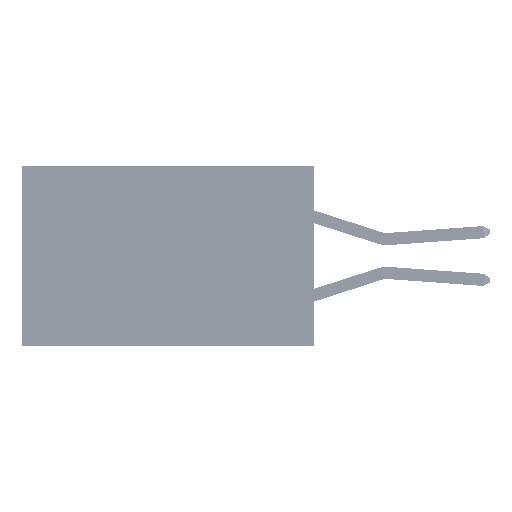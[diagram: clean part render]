
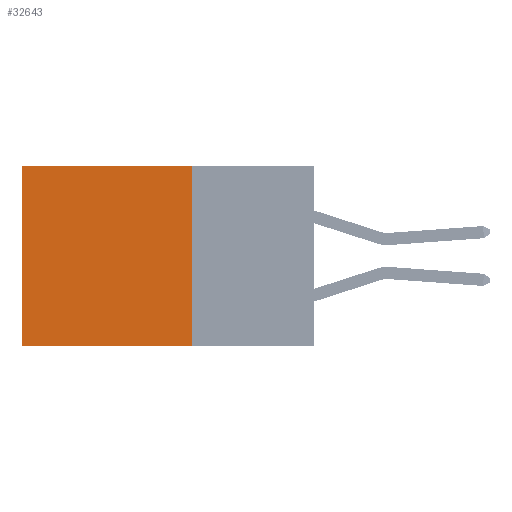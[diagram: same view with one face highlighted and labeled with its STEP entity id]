
A CAD part, left-side view. The second image highlights one B-rep face of the part: STEP entity #32643.
In plain terms, the highlighted planar face has unit normal (-1, 0, 0).
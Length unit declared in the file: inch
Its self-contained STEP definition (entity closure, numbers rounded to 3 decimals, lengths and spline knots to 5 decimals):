
#1590 = EDGE_CURVE ( 'NONE', #46278, #43713, #3092, .T. ) ;
#3092 = LINE ( 'NONE', #15803, #29588 ) ;
#3892 = FACE_OUTER_BOUND ( 'NONE', #48958, .T. ) ;
#6609 = DIRECTION ( 'NONE',  ( 0., 0., -1. ) ) ;
#9017 = VECTOR ( 'NONE', #17560, 39.37008 ) ;
#15061 = LINE ( 'NONE', #21394, #9017 ) ;
#15562 = DIRECTION ( 'NONE',  ( 0., 1., 0. ) ) ;
#15803 = CARTESIAN_POINT ( 'NONE',  ( 0.2875, 0.25, 0. ) ) ;
#15960 = CARTESIAN_POINT ( 'NONE',  ( 0.2875, 0.25, -0.37 ) ) ;
#17560 = DIRECTION ( 'NONE',  ( 0., 1., 0. ) ) ;
#19490 = DIRECTION ( 'NONE',  ( 0., 0., -1. ) ) ;
#20014 = ORIENTED_EDGE ( 'NONE', *, *, #42223, .T. ) ;
#20800 = VECTOR ( 'NONE', #15562, 39.37008 ) ;
#21354 = LINE ( 'NONE', #31228, #37404 ) ;
#21394 = CARTESIAN_POINT ( 'NONE',  ( 0.2875, 0.25, -0.37 ) ) ;
#27652 = CARTESIAN_POINT ( 'NONE',  ( 0.2875, 0.25, 0. ) ) ;
#29588 = VECTOR ( 'NONE', #38997, 39.37008 ) ;
#29955 = CARTESIAN_POINT ( 'NONE',  ( 0.2875, 0.6, 0. ) ) ;
#30036 = ORIENTED_EDGE ( 'NONE', *, *, #31015, .F. ) ;
#30327 = VERTEX_POINT ( 'NONE', #45468 ) ;
#31015 = EDGE_CURVE ( 'NONE', #43713, #30327, #15061, .T. ) ;
#31228 = CARTESIAN_POINT ( 'NONE',  ( 0.2875, 0.6, 0. ) ) ;
#32643 = ADVANCED_FACE ( 'NONE', ( #3892 ), #46275, .F. ) ;
#35157 = ORIENTED_EDGE ( 'NONE', *, *, #43025, .T. ) ;
#36860 = LINE ( 'NONE', #27652, #20800 ) ;
#37404 = VECTOR ( 'NONE', #19490, 39.37008 ) ;
#37827 = CARTESIAN_POINT ( 'NONE',  ( 0.2875, 0.25, 0. ) ) ;
#38997 = DIRECTION ( 'NONE',  ( 0., 0., -1. ) ) ;
#39269 = VERTEX_POINT ( 'NONE', #29955 ) ;
#42223 = EDGE_CURVE ( 'NONE', #46278, #39269, #36860, .T. ) ;
#43025 = EDGE_CURVE ( 'NONE', #39269, #30327, #21354, .T. ) ;
#43713 = VERTEX_POINT ( 'NONE', #15960 ) ;
#45468 = CARTESIAN_POINT ( 'NONE',  ( 0.2875, 0.6, -0.37 ) ) ;
#46275 = PLANE ( 'NONE',  #50115 ) ;
#46278 = VERTEX_POINT ( 'NONE', #49216 ) ;
#46840 = ORIENTED_EDGE ( 'NONE', *, *, #1590, .F. ) ;
#48958 = EDGE_LOOP ( 'NONE', ( #35157, #30036, #46840, #20014 ) ) ;
#49216 = CARTESIAN_POINT ( 'NONE',  ( 0.2875, 0.25, 0. ) ) ;
#50115 = AXIS2_PLACEMENT_3D ( 'NONE', #37827, #50268, #6609 ) ;
#50268 = DIRECTION ( 'NONE',  ( 1., 0., 0. ) ) ;
